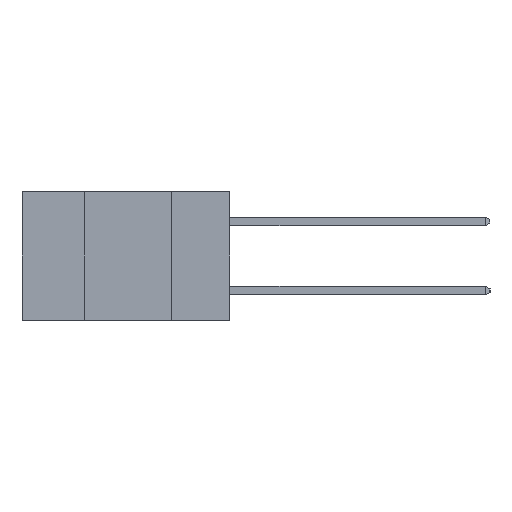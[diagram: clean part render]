
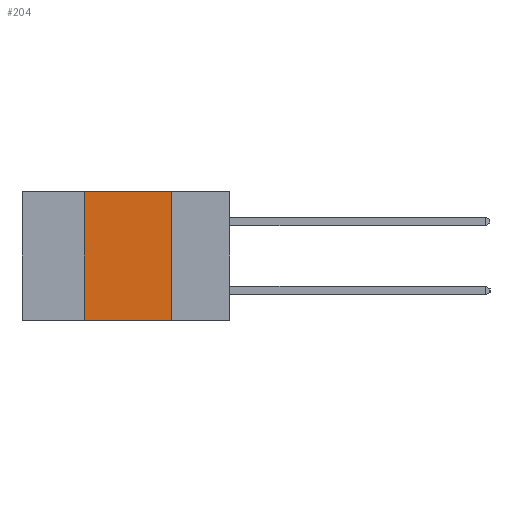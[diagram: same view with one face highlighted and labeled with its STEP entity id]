
A CAD part, left-side view. The second image highlights one B-rep face of the part: STEP entity #204.
In plain terms, the highlighted planar face has unit normal (-1, 0, 0).
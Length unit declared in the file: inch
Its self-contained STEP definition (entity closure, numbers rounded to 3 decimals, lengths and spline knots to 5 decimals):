
#177 = EDGE_CURVE ( 'NONE', #818, #2711, #6471, .T. ) ;
#204 = ADVANCED_FACE ( 'NONE', ( #14825 ), #18143, .F. ) ;
#818 = VERTEX_POINT ( 'NONE', #4067 ) ;
#830 = DIRECTION ( 'NONE',  ( 0., -1., 0. ) ) ;
#2070 = ORIENTED_EDGE ( 'NONE', *, *, #14485, .T. ) ;
#2711 = VERTEX_POINT ( 'NONE', #11146 ) ;
#4067 = CARTESIAN_POINT ( 'NONE',  ( 0., 0.42, -0.37 ) ) ;
#4524 = CARTESIAN_POINT ( 'NONE',  ( 0., 0.17, 0. ) ) ;
#5187 = VECTOR ( 'NONE', #830, 39.37008 ) ;
#5615 = EDGE_CURVE ( 'NONE', #10510, #15573, #9322, .T. ) ;
#6471 = LINE ( 'NONE', #14849, #18374 ) ;
#7231 = DIRECTION ( 'NONE',  ( 0., 0., 1. ) ) ;
#9124 = ORIENTED_EDGE ( 'NONE', *, *, #177, .F. ) ;
#9322 = LINE ( 'NONE', #17260, #17030 ) ;
#10209 = DIRECTION ( 'NONE',  ( 0., 0., -1. ) ) ;
#10510 = VERTEX_POINT ( 'NONE', #4524 ) ;
#10808 = CARTESIAN_POINT ( 'NONE',  ( 0., 0.17, -0.37 ) ) ;
#11146 = CARTESIAN_POINT ( 'NONE',  ( 0., 0.42, 0. ) ) ;
#12226 = DIRECTION ( 'NONE',  ( 0., -1., 0. ) ) ;
#12287 = DIRECTION ( 'NONE',  ( 1., 0., 0. ) ) ;
#14485 = EDGE_CURVE ( 'NONE', #818, #15573, #19845, .T. ) ;
#14825 = FACE_OUTER_BOUND ( 'NONE', #18469, .T. ) ;
#14849 = CARTESIAN_POINT ( 'NONE',  ( 0., 0.42, -0.37 ) ) ;
#14956 = CARTESIAN_POINT ( 'NONE',  ( 0., 0.6, 0. ) ) ;
#15573 = VERTEX_POINT ( 'NONE', #10808 ) ;
#15897 = ORIENTED_EDGE ( 'NONE', *, *, #5615, .F. ) ;
#16358 = AXIS2_PLACEMENT_3D ( 'NONE', #14956, #12287, #10209 ) ;
#16688 = LINE ( 'NONE', #19621, #5187 ) ;
#16821 = CARTESIAN_POINT ( 'NONE',  ( 0., 0.6, -0.37 ) ) ;
#17030 = VECTOR ( 'NONE', #18775, 39.37008 ) ;
#17260 = CARTESIAN_POINT ( 'NONE',  ( 0., 0.17, -0.37 ) ) ;
#17826 = ORIENTED_EDGE ( 'NONE', *, *, #18525, .F. ) ;
#18143 = PLANE ( 'NONE',  #16358 ) ;
#18374 = VECTOR ( 'NONE', #7231, 39.37008 ) ;
#18469 = EDGE_LOOP ( 'NONE', ( #15897, #17826, #9124, #2070 ) ) ;
#18525 = EDGE_CURVE ( 'NONE', #2711, #10510, #16688, .T. ) ;
#18775 = DIRECTION ( 'NONE',  ( 0., 0., -1. ) ) ;
#19371 = VECTOR ( 'NONE', #12226, 39.37008 ) ;
#19621 = CARTESIAN_POINT ( 'NONE',  ( 0., 0.6, 0. ) ) ;
#19845 = LINE ( 'NONE', #16821, #19371 ) ;
